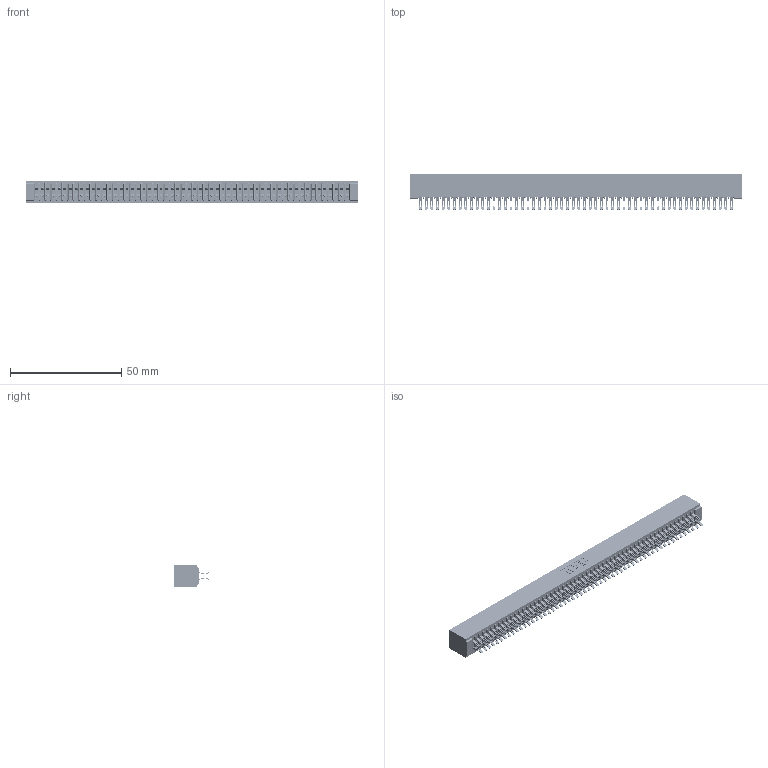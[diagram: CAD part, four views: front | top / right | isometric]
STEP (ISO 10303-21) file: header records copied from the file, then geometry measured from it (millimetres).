
FILE_DESCRIPTION (( 'STEP AP203' ), '1' );
FILE_NAME ('341-112-555-201.STEP', '2018-08-08T13:12:12', ( '' ), ( '' ), 'SwSTEP 2.0', 'SolidWorks 2016', '' );
FILE_SCHEMA (( 'CONFIG_CONTROL_DESIGN' ));
Length unit declared in the file: inch
Products named in the file (3): 341 Part_No Mounting Lugs; 341-292-001_341-292-155; 341-112-555-201
Assembly tree (113 placements, depth 2):
  341-112-555-201
    341 Part_No Mounting Lugs
    341-292-001_341-292-155  x112
Bounding box: 149.22 x 16.31 x 10.16 mm (x, y, z)
Volume: 11410.1 mm3; surface area: 22272.6 mm2
Topology: 113 solids, 113 shells, 8844 faces, 26444 edges, 17214 vertices
Faces by surface type: plane 4768, cylinder 3852, sphere 114, torus 110
Entity records: 66099 total; most frequent: CARTESIAN_POINT 11002, ORIENTED_EDGE 10924, DIRECTION 10656, EDGE_CURVE 5462, LINE 4416, VECTOR 4416, VERTEX_POINT 3450, AXIS2_PLACEMENT_3D 3120
